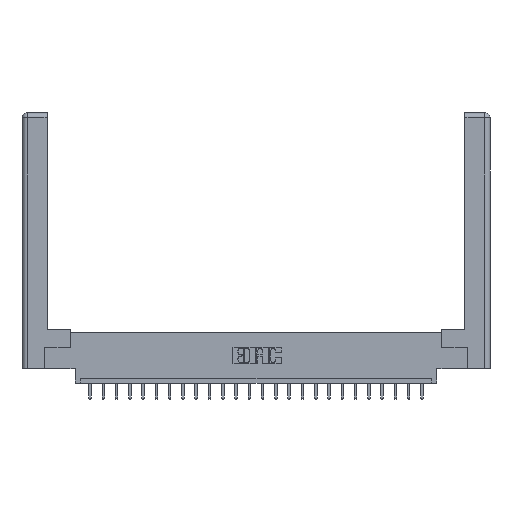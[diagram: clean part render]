
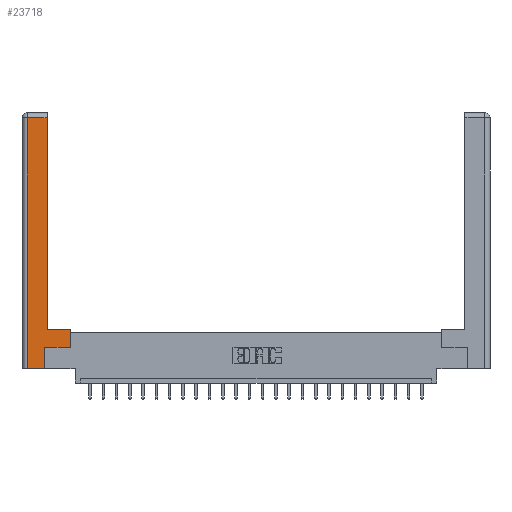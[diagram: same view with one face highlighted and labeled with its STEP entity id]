
A CAD part, top view. The second image highlights one B-rep face of the part: STEP entity #23718.
In plain terms, the highlighted planar face has unit normal (0, 0, 1).
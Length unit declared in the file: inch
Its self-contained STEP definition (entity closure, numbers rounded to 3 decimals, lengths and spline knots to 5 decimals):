
#82 = VERTEX_POINT ( 'NONE', #6117 ) ;
#214 = ORIENTED_EDGE ( 'NONE', *, *, #15800, .T. ) ;
#1102 = LINE ( 'NONE', #17809, #16703 ) ;
#1346 = CARTESIAN_POINT ( 'NONE',  ( 0., 0., 0. ) ) ;
#1601 = CARTESIAN_POINT ( 'NONE',  ( 0.0615, 0., 0. ) ) ;
#1686 = CARTESIAN_POINT ( 'NONE',  ( 0.565, 0.45, 0. ) ) ;
#2188 = CARTESIAN_POINT ( 'NONE',  ( 0.0615, 2.94, 0. ) ) ;
#2688 = CARTESIAN_POINT ( 'NONE',  ( 0.265, 0.245, 0. ) ) ;
#2856 = LINE ( 'NONE', #20438, #18474 ) ;
#3955 = VERTEX_POINT ( 'NONE', #6266 ) ;
#4307 = LINE ( 'NONE', #1601, #16988 ) ;
#4357 = VERTEX_POINT ( 'NONE', #2188 ) ;
#4429 = EDGE_CURVE ( 'NONE', #82, #4357, #20629, .T. ) ;
#4864 = LINE ( 'NONE', #22157, #17542 ) ;
#5083 = LINE ( 'NONE', #22406, #12427 ) ;
#5773 = DIRECTION ( 'NONE',  ( 0., 1., 0. ) ) ;
#5915 = EDGE_CURVE ( 'NONE', #3955, #13611, #1102, .T. ) ;
#6109 = CARTESIAN_POINT ( 'NONE',  ( 0.0615, 2.94, 0. ) ) ;
#6117 = CARTESIAN_POINT ( 'NONE',  ( 0.295, 2.94, 0. ) ) ;
#6266 = CARTESIAN_POINT ( 'NONE',  ( 0.265, 0.245, 0. ) ) ;
#7322 = DIRECTION ( 'NONE',  ( 0., 1., 0. ) ) ;
#8322 = DIRECTION ( 'NONE',  ( 1., 0., 0. ) ) ;
#8627 = CARTESIAN_POINT ( 'NONE',  ( 0.0615, 0., 0. ) ) ;
#9970 = LINE ( 'NONE', #1686, #22004 ) ;
#10204 = CARTESIAN_POINT ( 'NONE',  ( 0.565, 0.45, 0. ) ) ;
#10949 = DIRECTION ( 'NONE',  ( 0., 0., -1. ) ) ;
#11167 = DIRECTION ( 'NONE',  ( 1., 0., 0. ) ) ;
#11782 = DIRECTION ( 'NONE',  ( -1., 0., 0. ) ) ;
#11848 = VERTEX_POINT ( 'NONE', #15332 ) ;
#11914 = ORIENTED_EDGE ( 'NONE', *, *, #19463, .T. ) ;
#12427 = VECTOR ( 'NONE', #11167, 39.37008 ) ;
#13093 = ORIENTED_EDGE ( 'NONE', *, *, #17797, .T. ) ;
#13178 = ORIENTED_EDGE ( 'NONE', *, *, #14558, .T. ) ;
#13343 = CARTESIAN_POINT ( 'NONE',  ( 0.265, 0., 0. ) ) ;
#13611 = VERTEX_POINT ( 'NONE', #20819 ) ;
#13700 = EDGE_LOOP ( 'NONE', ( #214, #14068, #23140, #13093, #16997, #18072, #13178, #11914 ) ) ;
#14068 = ORIENTED_EDGE ( 'NONE', *, *, #4429, .T. ) ;
#14519 = DIRECTION ( 'NONE',  ( 0., -1., 0. ) ) ;
#14558 = EDGE_CURVE ( 'NONE', #13611, #22202, #9970, .T. ) ;
#14927 = VERTEX_POINT ( 'NONE', #8627 ) ;
#15206 = VECTOR ( 'NONE', #16120, 39.37008 ) ;
#15332 = CARTESIAN_POINT ( 'NONE',  ( 0.295, 0.45, 0. ) ) ;
#15537 = EDGE_CURVE ( 'NONE', #4357, #14927, #4307, .T. ) ;
#15624 = VECTOR ( 'NONE', #11782, 39.37008 ) ;
#15794 = LINE ( 'NONE', #2688, #15206 ) ;
#15800 = EDGE_CURVE ( 'NONE', #11848, #82, #2856, .T. ) ;
#16120 = DIRECTION ( 'NONE',  ( 0., 1., 0. ) ) ;
#16307 = EDGE_CURVE ( 'NONE', #18663, #3955, #15794, .T. ) ;
#16703 = VECTOR ( 'NONE', #8322, 39.37008 ) ;
#16988 = VECTOR ( 'NONE', #14519, 39.37008 ) ;
#16997 = ORIENTED_EDGE ( 'NONE', *, *, #16307, .T. ) ;
#17542 = VECTOR ( 'NONE', #24028, 39.37008 ) ;
#17797 = EDGE_CURVE ( 'NONE', #14927, #18663, #5083, .T. ) ;
#17809 = CARTESIAN_POINT ( 'NONE',  ( 0.565, 0.245, 0. ) ) ;
#18072 = ORIENTED_EDGE ( 'NONE', *, *, #5915, .T. ) ;
#18474 = VECTOR ( 'NONE', #5773, 39.37008 ) ;
#18545 = DIRECTION ( 'NONE',  ( -1., 0., 0. ) ) ;
#18663 = VERTEX_POINT ( 'NONE', #13343 ) ;
#19463 = EDGE_CURVE ( 'NONE', #22202, #11848, #4864, .T. ) ;
#20007 = FACE_OUTER_BOUND ( 'NONE', #13700, .T. ) ;
#20431 = PLANE ( 'NONE',  #22825 ) ;
#20438 = CARTESIAN_POINT ( 'NONE',  ( 0.295, 3., 0. ) ) ;
#20629 = LINE ( 'NONE', #6109, #15624 ) ;
#20819 = CARTESIAN_POINT ( 'NONE',  ( 0.565, 0.245, 0. ) ) ;
#22004 = VECTOR ( 'NONE', #7322, 39.37008 ) ;
#22157 = CARTESIAN_POINT ( 'NONE',  ( 0.295, 0.45, 0. ) ) ;
#22202 = VERTEX_POINT ( 'NONE', #10204 ) ;
#22406 = CARTESIAN_POINT ( 'NONE',  ( 0.265, 0., 0. ) ) ;
#22825 = AXIS2_PLACEMENT_3D ( 'NONE', #1346, #10949, #18545 ) ;
#23140 = ORIENTED_EDGE ( 'NONE', *, *, #15537, .T. ) ;
#23718 = ADVANCED_FACE ( 'NONE', ( #20007 ), #20431, .F. ) ;
#24028 = DIRECTION ( 'NONE',  ( -1., 0., 0. ) ) ;
